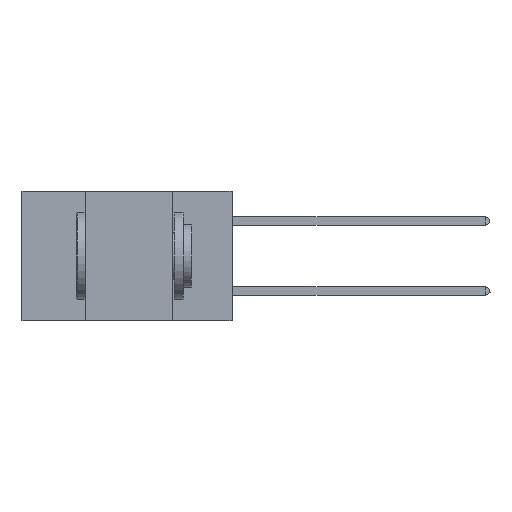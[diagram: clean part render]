
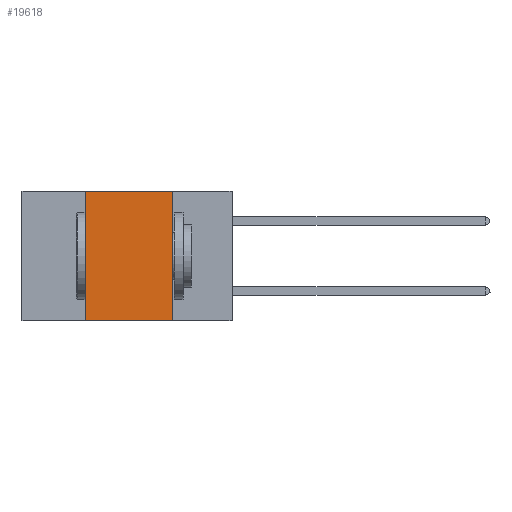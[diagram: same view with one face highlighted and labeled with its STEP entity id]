
A CAD part, left-side view. The second image highlights one B-rep face of the part: STEP entity #19618.
In plain terms, the highlighted planar face has unit normal (-1, 0, 0).
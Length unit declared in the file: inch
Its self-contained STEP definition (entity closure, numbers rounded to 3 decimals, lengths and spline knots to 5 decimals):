
#167 = ORIENTED_EDGE ( 'NONE', *, *, #7948, .T. ) ;
#4350 = VECTOR ( 'NONE', #19120, 39.37008 ) ;
#5196 = VERTEX_POINT ( 'NONE', #35745 ) ;
#5526 = EDGE_CURVE ( 'NONE', #41118, #5196, #44878, .T. ) ;
#6104 = DIRECTION ( 'NONE',  ( 0., 0., 1. ) ) ;
#6887 = VERTEX_POINT ( 'NONE', #45401 ) ;
#7095 = CARTESIAN_POINT ( 'NONE',  ( 0., 0.42, 0. ) ) ;
#7948 = EDGE_CURVE ( 'NONE', #6887, #5196, #23593, .T. ) ;
#8591 = VECTOR ( 'NONE', #18786, 39.37008 ) ;
#9369 = EDGE_CURVE ( 'NONE', #43749, #41118, #18555, .T. ) ;
#9508 = CARTESIAN_POINT ( 'NONE',  ( 0., 0.17, 0. ) ) ;
#10847 = CARTESIAN_POINT ( 'NONE',  ( 0., 0.6, 0. ) ) ;
#15426 = EDGE_CURVE ( 'NONE', #6887, #43749, #40012, .T. ) ;
#18555 = LINE ( 'NONE', #32752, #8591 ) ;
#18786 = DIRECTION ( 'NONE',  ( 0., -1., 0. ) ) ;
#19120 = DIRECTION ( 'NONE',  ( 0., -1., 0. ) ) ;
#19542 = CARTESIAN_POINT ( 'NONE',  ( 0., 0.42, 0. ) ) ;
#19618 = ADVANCED_FACE ( 'NONE', ( #45232 ), #27939, .F. ) ;
#23593 = LINE ( 'NONE', #36449, #4350 ) ;
#24206 = CARTESIAN_POINT ( 'NONE',  ( 0., 0.17, 0. ) ) ;
#25402 = AXIS2_PLACEMENT_3D ( 'NONE', #10847, #35128, #28088 ) ;
#27013 = ORIENTED_EDGE ( 'NONE', *, *, #5526, .F. ) ;
#27939 = PLANE ( 'NONE',  #25402 ) ;
#28088 = DIRECTION ( 'NONE',  ( 0., 0., -1. ) ) ;
#32752 = CARTESIAN_POINT ( 'NONE',  ( 0., 0.6, 0. ) ) ;
#33421 = DIRECTION ( 'NONE',  ( 0., 0., -1. ) ) ;
#35128 = DIRECTION ( 'NONE',  ( 1., 0., 0. ) ) ;
#35745 = CARTESIAN_POINT ( 'NONE',  ( 0., 0.17, -0.37 ) ) ;
#36449 = CARTESIAN_POINT ( 'NONE',  ( 0., 0.6, -0.37 ) ) ;
#37002 = ORIENTED_EDGE ( 'NONE', *, *, #9369, .F. ) ;
#37834 = VECTOR ( 'NONE', #6104, 39.37008 ) ;
#38542 = EDGE_LOOP ( 'NONE', ( #27013, #37002, #42633, #167 ) ) ;
#40012 = LINE ( 'NONE', #19542, #37834 ) ;
#41118 = VERTEX_POINT ( 'NONE', #9508 ) ;
#42633 = ORIENTED_EDGE ( 'NONE', *, *, #15426, .F. ) ;
#43187 = VECTOR ( 'NONE', #33421, 39.37008 ) ;
#43749 = VERTEX_POINT ( 'NONE', #7095 ) ;
#44878 = LINE ( 'NONE', #24206, #43187 ) ;
#45232 = FACE_OUTER_BOUND ( 'NONE', #38542, .T. ) ;
#45401 = CARTESIAN_POINT ( 'NONE',  ( 0., 0.42, -0.37 ) ) ;
